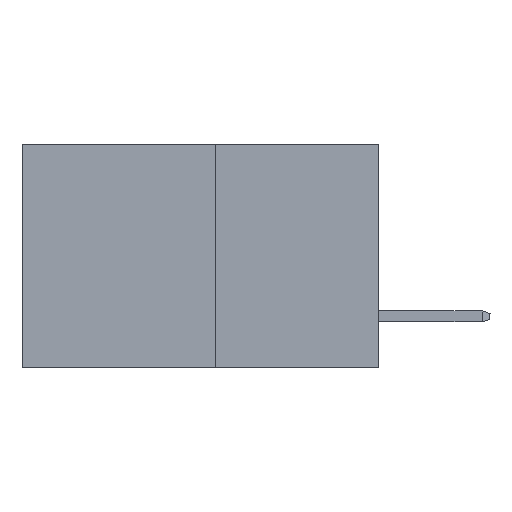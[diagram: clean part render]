
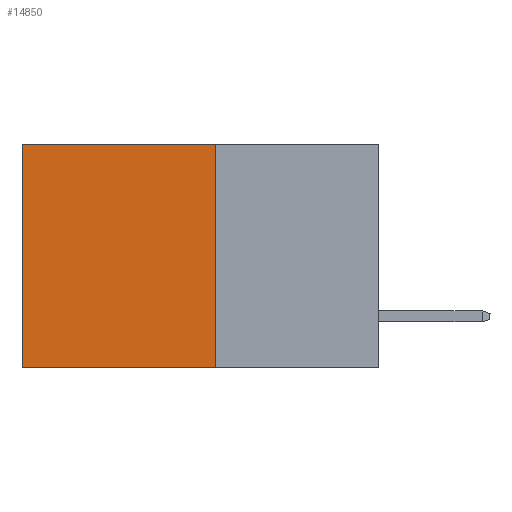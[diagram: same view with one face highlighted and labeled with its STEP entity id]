
A CAD part, left-side view. The second image highlights one B-rep face of the part: STEP entity #14850.
In plain terms, the highlighted planar face has unit normal (-1, 0, 0).
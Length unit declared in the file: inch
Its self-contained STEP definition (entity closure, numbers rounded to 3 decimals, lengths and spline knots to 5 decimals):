
#13 = CARTESIAN_POINT ( 'NONE',  ( 0.277, 0.27, 0. ) ) ;
#268 = CARTESIAN_POINT ( 'NONE',  ( 0.277, 0.59, -0.37 ) ) ;
#350 = EDGE_CURVE ( 'NONE', #4148, #15983, #5072, .T. ) ;
#671 = EDGE_CURVE ( 'NONE', #2918, #12785, #2838, .T. ) ;
#1798 = EDGE_LOOP ( 'NONE', ( #13864, #2691, #3494, #2776 ) ) ;
#1868 = VECTOR ( 'NONE', #6081, 39.37008 ) ;
#2504 = CARTESIAN_POINT ( 'NONE',  ( 0.277, 0.59, 0. ) ) ;
#2691 = ORIENTED_EDGE ( 'NONE', *, *, #11715, .F. ) ;
#2776 = ORIENTED_EDGE ( 'NONE', *, *, #16408, .T. ) ;
#2838 = LINE ( 'NONE', #15004, #6511 ) ;
#2918 = VERTEX_POINT ( 'NONE', #8346 ) ;
#2942 = CARTESIAN_POINT ( 'NONE',  ( 0.277, 0.27, -0.37 ) ) ;
#3494 = ORIENTED_EDGE ( 'NONE', *, *, #671, .F. ) ;
#4148 = VERTEX_POINT ( 'NONE', #2504 ) ;
#5072 = LINE ( 'NONE', #268, #13346 ) ;
#5304 = DIRECTION ( 'NONE',  ( 0., 0., -1. ) ) ;
#6081 = DIRECTION ( 'NONE',  ( 0., 1., 0. ) ) ;
#6511 = VECTOR ( 'NONE', #5304, 39.37008 ) ;
#7024 = DIRECTION ( 'NONE',  ( 0., 0., -1. ) ) ;
#8277 = LINE ( 'NONE', #13, #12408 ) ;
#8346 = CARTESIAN_POINT ( 'NONE',  ( 0.277, 0.27, 0. ) ) ;
#9042 = AXIS2_PLACEMENT_3D ( 'NONE', #11663, #16244, #7024 ) ;
#9608 = FACE_OUTER_BOUND ( 'NONE', #1798, .T. ) ;
#11663 = CARTESIAN_POINT ( 'NONE',  ( 0.277, 0.27, -0.37 ) ) ;
#11715 = EDGE_CURVE ( 'NONE', #12785, #15983, #17872, .T. ) ;
#12408 = VECTOR ( 'NONE', #12547, 39.37008 ) ;
#12547 = DIRECTION ( 'NONE',  ( 0., 1., 0. ) ) ;
#12785 = VERTEX_POINT ( 'NONE', #15661 ) ;
#13346 = VECTOR ( 'NONE', #14979, 39.37008 ) ;
#13864 = ORIENTED_EDGE ( 'NONE', *, *, #350, .T. ) ;
#14615 = CARTESIAN_POINT ( 'NONE',  ( 0.277, 0.59, -0.37 ) ) ;
#14713 = PLANE ( 'NONE',  #9042 ) ;
#14850 = ADVANCED_FACE ( 'NONE', ( #9608 ), #14713, .F. ) ;
#14979 = DIRECTION ( 'NONE',  ( 0., 0., -1. ) ) ;
#15004 = CARTESIAN_POINT ( 'NONE',  ( 0.277, 0.27, -0.37 ) ) ;
#15661 = CARTESIAN_POINT ( 'NONE',  ( 0.277, 0.27, -0.37 ) ) ;
#15983 = VERTEX_POINT ( 'NONE', #14615 ) ;
#16244 = DIRECTION ( 'NONE',  ( 1., 0., 0. ) ) ;
#16408 = EDGE_CURVE ( 'NONE', #2918, #4148, #8277, .T. ) ;
#17872 = LINE ( 'NONE', #2942, #1868 ) ;
